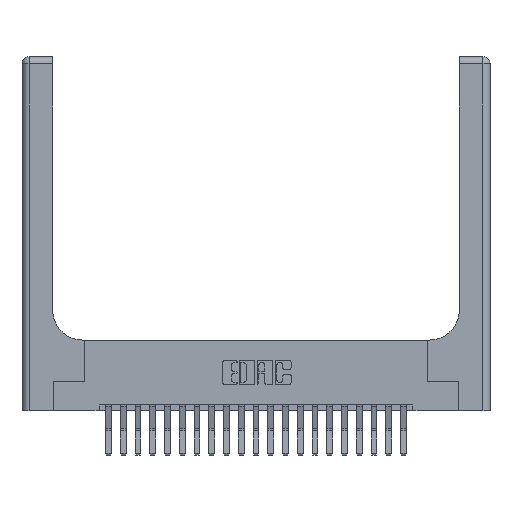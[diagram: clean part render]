
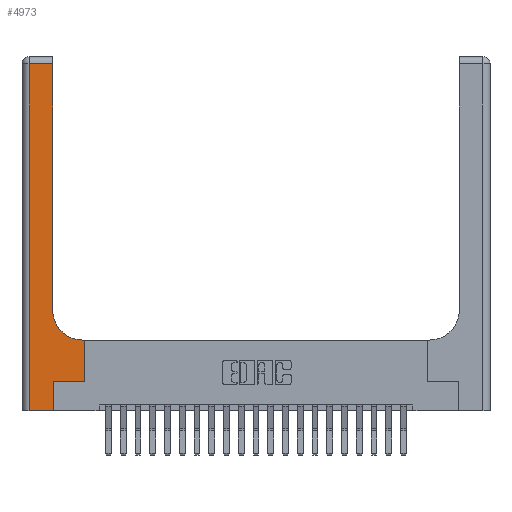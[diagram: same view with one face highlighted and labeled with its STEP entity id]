
A CAD part, top view. The second image highlights one B-rep face of the part: STEP entity #4973.
In plain terms, the highlighted planar face has unit normal (0, 0, 1).
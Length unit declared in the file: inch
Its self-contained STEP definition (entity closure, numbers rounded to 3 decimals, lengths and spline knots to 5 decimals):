
#137 = AXIS2_PLACEMENT_3D ( 'NONE', #19330, #17644, #2217 ) ;
#288 = VERTEX_POINT ( 'NONE', #7039 ) ;
#606 = CARTESIAN_POINT ( 'NONE',  ( 0.06, 0., 0.37 ) ) ;
#922 = CARTESIAN_POINT ( 'NONE',  ( 0.265, 0.25, 0.37 ) ) ;
#1095 = LINE ( 'NONE', #6596, #19168 ) ;
#1312 = EDGE_CURVE ( 'NONE', #288, #17060, #7760, .T. ) ;
#2048 = ORIENTED_EDGE ( 'NONE', *, *, #11060, .T. ) ;
#2141 = DIRECTION ( 'NONE',  ( 1., 0., 0. ) ) ;
#2217 = DIRECTION ( 'NONE',  ( -1., 0., 0. ) ) ;
#2404 = DIRECTION ( 'NONE',  ( 0., 1., 0. ) ) ;
#2415 = VECTOR ( 'NONE', #16637, 39.37008 ) ;
#2486 = VERTEX_POINT ( 'NONE', #21277 ) ;
#2994 = CARTESIAN_POINT ( 'NONE',  ( 0., 0., 0.37 ) ) ;
#3207 = CIRCLE ( 'NONE', #15780, 0.25 ) ;
#4085 = LINE ( 'NONE', #10956, #5365 ) ;
#4572 = DIRECTION ( 'NONE',  ( 1., 0., 0. ) ) ;
#4851 = VERTEX_POINT ( 'NONE', #9079 ) ;
#4973 = ADVANCED_FACE ( 'NONE', ( #21018 ), #5605, .F. ) ;
#5300 = CARTESIAN_POINT ( 'NONE',  ( 0.26, 0.85, 0.37 ) ) ;
#5365 = VECTOR ( 'NONE', #2404, 39.37008 ) ;
#5605 = PLANE ( 'NONE',  #137 ) ;
#6258 = CARTESIAN_POINT ( 'NONE',  ( 0.265, 0.25, 0.37 ) ) ;
#6270 = EDGE_CURVE ( 'NONE', #4851, #14463, #16174, .T. ) ;
#6382 = LINE ( 'NONE', #2994, #19466 ) ;
#6433 = CARTESIAN_POINT ( 'NONE',  ( 0.265, 0., 0.37 ) ) ;
#6596 = CARTESIAN_POINT ( 'NONE',  ( 0., 2.94, 0.37 ) ) ;
#7039 = CARTESIAN_POINT ( 'NONE',  ( 0.06, 2.94, 0.37 ) ) ;
#7278 = EDGE_CURVE ( 'NONE', #2486, #14377, #3207, .T. ) ;
#7760 = LINE ( 'NONE', #9220, #19857 ) ;
#9079 = CARTESIAN_POINT ( 'NONE',  ( 0.528, 0.25, 0.37 ) ) ;
#9220 = CARTESIAN_POINT ( 'NONE',  ( 0.06, 3., 0.37 ) ) ;
#9556 = DIRECTION ( 'NONE',  ( 0., -1., 0. ) ) ;
#9962 = DIRECTION ( 'NONE',  ( -1., 0., 0. ) ) ;
#10548 = VERTEX_POINT ( 'NONE', #922 ) ;
#10956 = CARTESIAN_POINT ( 'NONE',  ( 0.26, 3., 0.37 ) ) ;
#11060 = EDGE_CURVE ( 'NONE', #14463, #2486, #16304, .T. ) ;
#11881 = VERTEX_POINT ( 'NONE', #6433 ) ;
#12920 = CARTESIAN_POINT ( 'NONE',  ( 0.26, 0.6, 0.37 ) ) ;
#12943 = ORIENTED_EDGE ( 'NONE', *, *, #1312, .T. ) ;
#12998 = LINE ( 'NONE', #6258, #16100 ) ;
#13011 = VECTOR ( 'NONE', #14488, 39.37008 ) ;
#13784 = ORIENTED_EDGE ( 'NONE', *, *, #6270, .T. ) ;
#13857 = VERTEX_POINT ( 'NONE', #19678 ) ;
#14245 = EDGE_CURVE ( 'NONE', #10548, #4851, #12998, .T. ) ;
#14377 = VERTEX_POINT ( 'NONE', #5300 ) ;
#14463 = VERTEX_POINT ( 'NONE', #21614 ) ;
#14488 = DIRECTION ( 'NONE',  ( -1., 0., 0. ) ) ;
#15015 = DIRECTION ( 'NONE',  ( 0., 1., 0. ) ) ;
#15633 = ORIENTED_EDGE ( 'NONE', *, *, #14245, .T. ) ;
#15651 = DIRECTION ( 'NONE',  ( 0., 0., -1. ) ) ;
#15780 = AXIS2_PLACEMENT_3D ( 'NONE', #17572, #15651, #2141 ) ;
#16084 = ORIENTED_EDGE ( 'NONE', *, *, #20009, .T. ) ;
#16100 = VECTOR ( 'NONE', #20388, 39.37008 ) ;
#16174 = LINE ( 'NONE', #18318, #2415 ) ;
#16304 = LINE ( 'NONE', #12920, #13011 ) ;
#16618 = LINE ( 'NONE', #22011, #20137 ) ;
#16637 = DIRECTION ( 'NONE',  ( 0., 1., 0. ) ) ;
#17060 = VERTEX_POINT ( 'NONE', #606 ) ;
#17115 = EDGE_CURVE ( 'NONE', #14377, #13857, #4085, .T. ) ;
#17149 = ORIENTED_EDGE ( 'NONE', *, *, #21405, .T. ) ;
#17291 = ORIENTED_EDGE ( 'NONE', *, *, #7278, .T. ) ;
#17572 = CARTESIAN_POINT ( 'NONE',  ( 0.51, 0.85, 0.37 ) ) ;
#17644 = DIRECTION ( 'NONE',  ( 0., 0., -1. ) ) ;
#18132 = EDGE_CURVE ( 'NONE', #11881, #10548, #16618, .T. ) ;
#18215 = ORIENTED_EDGE ( 'NONE', *, *, #18132, .T. ) ;
#18318 = CARTESIAN_POINT ( 'NONE',  ( 0.528, 0.25, 0.37 ) ) ;
#19168 = VECTOR ( 'NONE', #9962, 39.37008 ) ;
#19330 = CARTESIAN_POINT ( 'NONE',  ( 0., 3., 0.37 ) ) ;
#19466 = VECTOR ( 'NONE', #4572, 39.37008 ) ;
#19678 = CARTESIAN_POINT ( 'NONE',  ( 0.26, 2.94, 0.37 ) ) ;
#19857 = VECTOR ( 'NONE', #9556, 39.37008 ) ;
#20009 = EDGE_CURVE ( 'NONE', #17060, #11881, #6382, .T. ) ;
#20137 = VECTOR ( 'NONE', #15015, 39.37008 ) ;
#20153 = EDGE_LOOP ( 'NONE', ( #22149, #17149, #12943, #16084, #18215, #15633, #13784, #2048, #17291 ) ) ;
#20388 = DIRECTION ( 'NONE',  ( 1., 0., 0. ) ) ;
#21018 = FACE_OUTER_BOUND ( 'NONE', #20153, .T. ) ;
#21277 = CARTESIAN_POINT ( 'NONE',  ( 0.51, 0.6, 0.37 ) ) ;
#21405 = EDGE_CURVE ( 'NONE', #13857, #288, #1095, .T. ) ;
#21614 = CARTESIAN_POINT ( 'NONE',  ( 0.528, 0.6, 0.37 ) ) ;
#22011 = CARTESIAN_POINT ( 'NONE',  ( 0.265, 0., 0.37 ) ) ;
#22149 = ORIENTED_EDGE ( 'NONE', *, *, #17115, .T. ) ;
